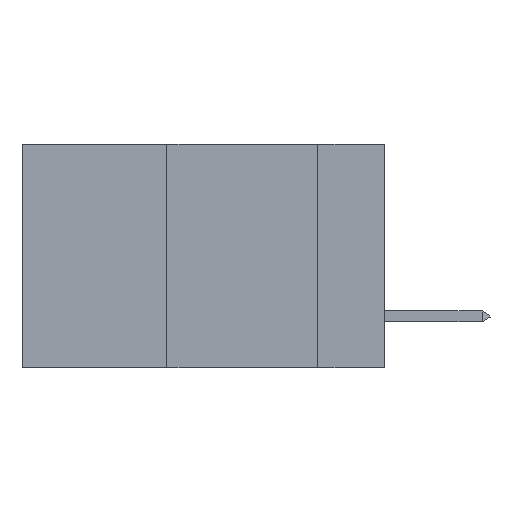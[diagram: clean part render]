
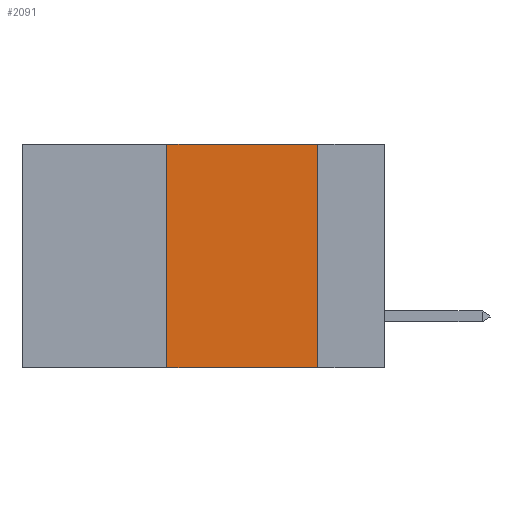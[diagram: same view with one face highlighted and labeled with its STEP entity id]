
A CAD part, left-side view. The second image highlights one B-rep face of the part: STEP entity #2091.
In plain terms, the highlighted planar face has unit normal (-1, 0, 0).
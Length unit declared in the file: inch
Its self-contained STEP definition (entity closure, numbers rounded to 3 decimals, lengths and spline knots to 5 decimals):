
#2091 = ADVANCED_FACE ( 'NONE', ( #27480 ), #4044, .F. ) ;
#3196 = LINE ( 'NONE', #4079, #14635 ) ;
#3436 = EDGE_CURVE ( 'NONE', #30211, #30998, #16959, .T. ) ;
#4044 = PLANE ( 'NONE',  #29291 ) ;
#4079 = CARTESIAN_POINT ( 'NONE',  ( 0., 0.11, 0. ) ) ;
#5104 = CARTESIAN_POINT ( 'NONE',  ( 0., 0.6, 0. ) ) ;
#5527 = DIRECTION ( 'NONE',  ( 1., 0., 0. ) ) ;
#6867 = CARTESIAN_POINT ( 'NONE',  ( 0., 0.11, 0. ) ) ;
#7613 = ORIENTED_EDGE ( 'NONE', *, *, #16846, .F. ) ;
#7718 = VERTEX_POINT ( 'NONE', #29700 ) ;
#8233 = CARTESIAN_POINT ( 'NONE',  ( 0., 0.6, 0. ) ) ;
#8507 = DIRECTION ( 'NONE',  ( 0., 0., 1. ) ) ;
#8923 = VECTOR ( 'NONE', #24087, 39.37008 ) ;
#9091 = DIRECTION ( 'NONE',  ( 0., 0., -1. ) ) ;
#11991 = DIRECTION ( 'NONE',  ( 0., 0., -1. ) ) ;
#13127 = DIRECTION ( 'NONE',  ( 0., -1., 0. ) ) ;
#14162 = EDGE_CURVE ( 'NONE', #7718, #25753, #19431, .T. ) ;
#14205 = ORIENTED_EDGE ( 'NONE', *, *, #3436, .T. ) ;
#14635 = VECTOR ( 'NONE', #9091, 39.37008 ) ;
#15930 = LINE ( 'NONE', #20397, #20548 ) ;
#15968 = EDGE_CURVE ( 'NONE', #30211, #7718, #15930, .T. ) ;
#16607 = ORIENTED_EDGE ( 'NONE', *, *, #15968, .F. ) ;
#16846 = EDGE_CURVE ( 'NONE', #25753, #30998, #3196, .T. ) ;
#16959 = LINE ( 'NONE', #21293, #8923 ) ;
#17876 = CARTESIAN_POINT ( 'NONE',  ( 0., 0.11, -0.37 ) ) ;
#19431 = LINE ( 'NONE', #8233, #31772 ) ;
#20397 = CARTESIAN_POINT ( 'NONE',  ( 0., 0.36, 0. ) ) ;
#20548 = VECTOR ( 'NONE', #8507, 39.37008 ) ;
#21293 = CARTESIAN_POINT ( 'NONE',  ( 0., 0.6, -0.37 ) ) ;
#23146 = EDGE_LOOP ( 'NONE', ( #7613, #24442, #16607, #14205 ) ) ;
#24087 = DIRECTION ( 'NONE',  ( 0., -1., 0. ) ) ;
#24442 = ORIENTED_EDGE ( 'NONE', *, *, #14162, .F. ) ;
#25753 = VERTEX_POINT ( 'NONE', #6867 ) ;
#27480 = FACE_OUTER_BOUND ( 'NONE', #23146, .T. ) ;
#29291 = AXIS2_PLACEMENT_3D ( 'NONE', #5104, #5527, #11991 ) ;
#29545 = CARTESIAN_POINT ( 'NONE',  ( 0., 0.36, -0.37 ) ) ;
#29700 = CARTESIAN_POINT ( 'NONE',  ( 0., 0.36, 0. ) ) ;
#30211 = VERTEX_POINT ( 'NONE', #29545 ) ;
#30998 = VERTEX_POINT ( 'NONE', #17876 ) ;
#31772 = VECTOR ( 'NONE', #13127, 39.37008 ) ;
